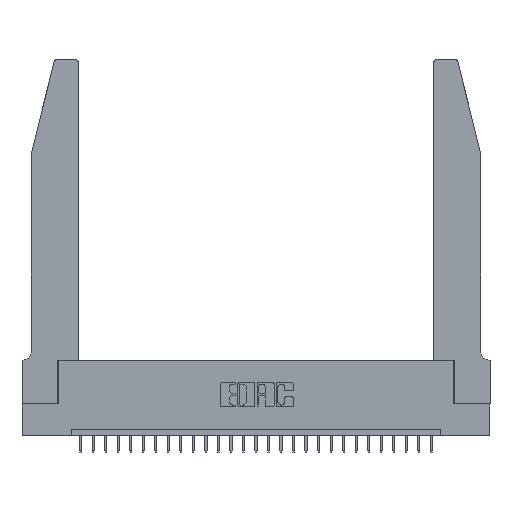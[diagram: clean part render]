
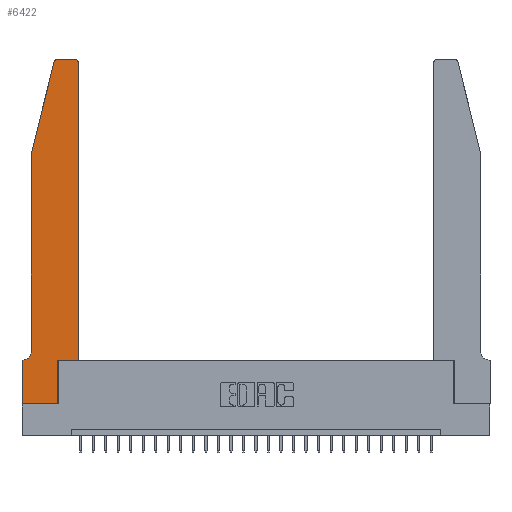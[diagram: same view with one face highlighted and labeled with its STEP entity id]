
A CAD part, top view. The second image highlights one B-rep face of the part: STEP entity #6422.
In plain terms, the highlighted planar face has unit normal (0, 0, 1).
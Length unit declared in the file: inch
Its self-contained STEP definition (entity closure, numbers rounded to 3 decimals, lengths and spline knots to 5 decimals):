
#43 = CARTESIAN_POINT ( 'NONE',  ( 0.284, 2.75, 0.37 ) ) ;
#1338 = CARTESIAN_POINT ( 'NONE',  ( 0.284, 2.72, 0.37 ) ) ;
#1784 = CARTESIAN_POINT ( 'NONE',  ( 0.4505, 0.35, 0.37 ) ) ;
#1848 = EDGE_CURVE ( 'NONE', #11211, #20339, #10559, .T. ) ;
#1943 = CARTESIAN_POINT ( 'NONE',  ( 0., 0.35, 0.37 ) ) ;
#1966 = ORIENTED_EDGE ( 'NONE', *, *, #23961, .T. ) ;
#2489 = LINE ( 'NONE', #11110, #4872 ) ;
#2505 = DIRECTION ( 'NONE',  ( 0., -1., 0. ) ) ;
#2798 = AXIS2_PLACEMENT_3D ( 'NONE', #1338, #20874, #18586 ) ;
#2863 = VERTEX_POINT ( 'NONE', #12236 ) ;
#3282 = CARTESIAN_POINT ( 'NONE',  ( 0., 0., 0.37 ) ) ;
#3474 = EDGE_CURVE ( 'NONE', #10262, #24170, #7941, .T. ) ;
#3846 = VERTEX_POINT ( 'NONE', #1943 ) ;
#4172 = EDGE_CURVE ( 'NONE', #20111, #6289, #21160, .T. ) ;
#4412 = CARTESIAN_POINT ( 'NONE',  ( 0.25487, 2.72718, 0.37 ) ) ;
#4756 = DIRECTION ( 'NONE',  ( 1., 0., 0. ) ) ;
#4872 = VECTOR ( 'NONE', #26770, 39.37008 ) ;
#5228 = VECTOR ( 'NONE', #18375, 39.37008 ) ;
#5407 = DIRECTION ( 'NONE',  ( 0., 0., 1. ) ) ;
#6154 = EDGE_CURVE ( 'NONE', #2863, #11211, #21781, .T. ) ;
#6250 = AXIS2_PLACEMENT_3D ( 'NONE', #9706, #5407, #9841 ) ;
#6289 = VERTEX_POINT ( 'NONE', #4412 ) ;
#6422 = ADVANCED_FACE ( 'NONE', ( #22765 ), #20629, .T. ) ;
#6442 = EDGE_CURVE ( 'NONE', #23848, #9819, #10280, .T. ) ;
#6770 = ORIENTED_EDGE ( 'NONE', *, *, #18428, .T. ) ;
#6891 = VECTOR ( 'NONE', #2505, 39.37008 ) ;
#7315 = LINE ( 'NONE', #24432, #7329 ) ;
#7329 = VECTOR ( 'NONE', #24561, 39.37008 ) ;
#7514 = ORIENTED_EDGE ( 'NONE', *, *, #6442, .T. ) ;
#7941 = LINE ( 'NONE', #21126, #22476 ) ;
#8034 = DIRECTION ( 'NONE',  ( 1., 0., 0. ) ) ;
#8208 = CARTESIAN_POINT ( 'NONE',  ( 0.0055, 0.42, 0.37 ) ) ;
#8848 = LINE ( 'NONE', #19895, #6891 ) ;
#8923 = EDGE_CURVE ( 'NONE', #20339, #3846, #11897, .T. ) ;
#9086 = EDGE_CURVE ( 'NONE', #23971, #10262, #14901, .T. ) ;
#9706 = CARTESIAN_POINT ( 'NONE',  ( 0., 0.35, 0.37 ) ) ;
#9819 = VERTEX_POINT ( 'NONE', #10394 ) ;
#9841 = DIRECTION ( 'NONE',  ( 1., 0., 0. ) ) ;
#10161 = VERTEX_POINT ( 'NONE', #22581 ) ;
#10210 = ORIENTED_EDGE ( 'NONE', *, *, #6154, .T. ) ;
#10262 = VERTEX_POINT ( 'NONE', #26313 ) ;
#10280 = LINE ( 'NONE', #1784, #23667 ) ;
#10394 = CARTESIAN_POINT ( 'NONE',  ( 0.4505, 2.72, 0.37 ) ) ;
#10417 = DIRECTION ( 'NONE',  ( 0., 1., 0. ) ) ;
#10559 = CIRCLE ( 'NONE', #15526, 0.07 ) ;
#11110 = CARTESIAN_POINT ( 'NONE',  ( 0.2605, 2.75, 0.37 ) ) ;
#11211 = VERTEX_POINT ( 'NONE', #24907 ) ;
#11298 = VECTOR ( 'NONE', #4756, 39.37008 ) ;
#11897 = LINE ( 'NONE', #24984, #5228 ) ;
#12236 = CARTESIAN_POINT ( 'NONE',  ( 0.0755, 2., 0.37 ) ) ;
#12287 = AXIS2_PLACEMENT_3D ( 'NONE', #23105, #20932, #8034 ) ;
#12736 = CARTESIAN_POINT ( 'NONE',  ( 0., 0., 0.37 ) ) ;
#12875 = DIRECTION ( 'NONE',  ( 0., -1., 0. ) ) ;
#13536 = EDGE_CURVE ( 'NONE', #10161, #20111, #2489, .T. ) ;
#13714 = CARTESIAN_POINT ( 'NONE',  ( 0.2865, 0.35, 0.37 ) ) ;
#13950 = EDGE_CURVE ( 'NONE', #24170, #23848, #26318, .T. ) ;
#14637 = ORIENTED_EDGE ( 'NONE', *, *, #9086, .T. ) ;
#14901 = LINE ( 'NONE', #12736, #16691 ) ;
#15106 = CARTESIAN_POINT ( 'NONE',  ( 0.4505, 0.35, 0.37 ) ) ;
#15526 = AXIS2_PLACEMENT_3D ( 'NONE', #8208, #25739, #16957 ) ;
#15692 = EDGE_LOOP ( 'NONE', ( #26170, #17819, #20235, #10210, #23374, #26345, #6770, #14637, #27040, #16558, #7514, #1966 ) ) ;
#16558 = ORIENTED_EDGE ( 'NONE', *, *, #13950, .T. ) ;
#16691 = VECTOR ( 'NONE', #18806, 39.37008 ) ;
#16921 = CARTESIAN_POINT ( 'NONE',  ( 0.0755, 2., 0.37 ) ) ;
#16957 = DIRECTION ( 'NONE',  ( -1., 0., 0. ) ) ;
#17615 = EDGE_CURVE ( 'NONE', #6289, #2863, #7315, .T. ) ;
#17819 = ORIENTED_EDGE ( 'NONE', *, *, #4172, .T. ) ;
#18375 = DIRECTION ( 'NONE',  ( -1., 0., 0. ) ) ;
#18428 = EDGE_CURVE ( 'NONE', #3846, #23971, #8848, .T. ) ;
#18586 = DIRECTION ( 'NONE',  ( 1., 0., 0. ) ) ;
#18806 = DIRECTION ( 'NONE',  ( 1., 0., 0. ) ) ;
#19895 = CARTESIAN_POINT ( 'NONE',  ( 0., 0., 0.37 ) ) ;
#19983 = CARTESIAN_POINT ( 'NONE',  ( 0.4505, 0.35, 0.37 ) ) ;
#20111 = VERTEX_POINT ( 'NONE', #43 ) ;
#20235 = ORIENTED_EDGE ( 'NONE', *, *, #17615, .T. ) ;
#20339 = VERTEX_POINT ( 'NONE', #25884 ) ;
#20629 = PLANE ( 'NONE',  #6250 ) ;
#20874 = DIRECTION ( 'NONE',  ( 0., 0., 1. ) ) ;
#20932 = DIRECTION ( 'NONE',  ( 0., 0., 1. ) ) ;
#21126 = CARTESIAN_POINT ( 'NONE',  ( 0.2865, 0.35, 0.37 ) ) ;
#21160 = CIRCLE ( 'NONE', #2798, 0.03 ) ;
#21461 = CIRCLE ( 'NONE', #12287, 0.03 ) ;
#21781 = LINE ( 'NONE', #16921, #23646 ) ;
#22476 = VECTOR ( 'NONE', #25594, 39.37008 ) ;
#22581 = CARTESIAN_POINT ( 'NONE',  ( 0.4205, 2.75, 0.37 ) ) ;
#22765 = FACE_OUTER_BOUND ( 'NONE', #15692, .T. ) ;
#23105 = CARTESIAN_POINT ( 'NONE',  ( 0.4205, 2.72, 0.37 ) ) ;
#23374 = ORIENTED_EDGE ( 'NONE', *, *, #1848, .T. ) ;
#23646 = VECTOR ( 'NONE', #12875, 39.37008 ) ;
#23667 = VECTOR ( 'NONE', #10417, 39.37008 ) ;
#23848 = VERTEX_POINT ( 'NONE', #15106 ) ;
#23961 = EDGE_CURVE ( 'NONE', #9819, #10161, #21461, .T. ) ;
#23971 = VERTEX_POINT ( 'NONE', #3282 ) ;
#24170 = VERTEX_POINT ( 'NONE', #13714 ) ;
#24432 = CARTESIAN_POINT ( 'NONE',  ( 0.0755, 2., 0.37 ) ) ;
#24561 = DIRECTION ( 'NONE',  ( -0.239, -0.971, 0. ) ) ;
#24907 = CARTESIAN_POINT ( 'NONE',  ( 0.0755, 0.42, 0.37 ) ) ;
#24984 = CARTESIAN_POINT ( 'NONE',  ( 0.0755, 0.35, 0.37 ) ) ;
#25594 = DIRECTION ( 'NONE',  ( 0., 1., 0. ) ) ;
#25739 = DIRECTION ( 'NONE',  ( 0., 0., -1. ) ) ;
#25884 = CARTESIAN_POINT ( 'NONE',  ( 0.0055, 0.35, 0.37 ) ) ;
#26170 = ORIENTED_EDGE ( 'NONE', *, *, #13536, .T. ) ;
#26313 = CARTESIAN_POINT ( 'NONE',  ( 0.2865, 0., 0.37 ) ) ;
#26318 = LINE ( 'NONE', #19983, #11298 ) ;
#26345 = ORIENTED_EDGE ( 'NONE', *, *, #8923, .T. ) ;
#26770 = DIRECTION ( 'NONE',  ( -1., 0., 0. ) ) ;
#27040 = ORIENTED_EDGE ( 'NONE', *, *, #3474, .T. ) ;
